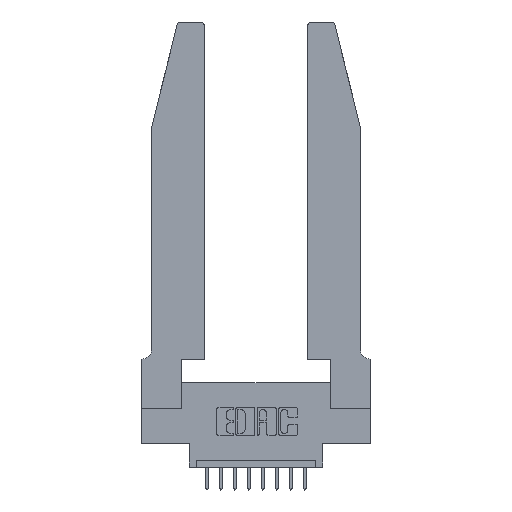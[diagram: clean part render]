
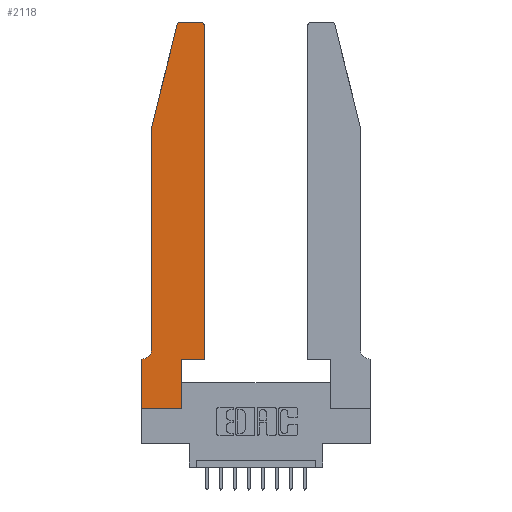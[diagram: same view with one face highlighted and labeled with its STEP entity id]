
A CAD part, top view. The second image highlights one B-rep face of the part: STEP entity #2118.
In plain terms, the highlighted planar face has unit normal (0, 0, 1).
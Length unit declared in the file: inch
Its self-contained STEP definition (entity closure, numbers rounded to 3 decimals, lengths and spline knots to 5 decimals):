
#182 = VERTEX_POINT ( 'NONE', #15368 ) ;
#187 = CARTESIAN_POINT ( 'NONE',  ( 0.284, 2.75, 0.37 ) ) ;
#546 = ORIENTED_EDGE ( 'NONE', *, *, #5395, .T. ) ;
#614 = CARTESIAN_POINT ( 'NONE',  ( 0., 0., 0.37 ) ) ;
#864 = VECTOR ( 'NONE', #15507, 39.37008 ) ;
#1088 = CARTESIAN_POINT ( 'NONE',  ( 0.2865, 0.35, 0.37 ) ) ;
#1105 = EDGE_CURVE ( 'NONE', #13346, #3585, #8174, .T. ) ;
#1202 = ORIENTED_EDGE ( 'NONE', *, *, #1105, .T. ) ;
#1531 = CARTESIAN_POINT ( 'NONE',  ( 0.0055, 0.42, 0.37 ) ) ;
#1691 = DIRECTION ( 'NONE',  ( 0., -1., 0. ) ) ;
#1773 = ORIENTED_EDGE ( 'NONE', *, *, #5691, .T. ) ;
#1904 = CARTESIAN_POINT ( 'NONE',  ( 0.4505, 0.35, 0.37 ) ) ;
#2008 = ORIENTED_EDGE ( 'NONE', *, *, #8542, .T. ) ;
#2118 = ADVANCED_FACE ( 'NONE', ( #8539 ), #2767, .T. ) ;
#2125 = CARTESIAN_POINT ( 'NONE',  ( 0.0755, 0.42, 0.37 ) ) ;
#2195 = LINE ( 'NONE', #2570, #8822 ) ;
#2570 = CARTESIAN_POINT ( 'NONE',  ( 0.0755, 2., 0.37 ) ) ;
#2637 = ORIENTED_EDGE ( 'NONE', *, *, #12434, .T. ) ;
#2767 = PLANE ( 'NONE',  #9166 ) ;
#3096 = VECTOR ( 'NONE', #4385, 39.37008 ) ;
#3184 = CIRCLE ( 'NONE', #5823, 0.03 ) ;
#3265 = CARTESIAN_POINT ( 'NONE',  ( 0.4505, 0.35, 0.37 ) ) ;
#3495 = LINE ( 'NONE', #8491, #9181 ) ;
#3585 = VERTEX_POINT ( 'NONE', #9422 ) ;
#3664 = EDGE_LOOP ( 'NONE', ( #3748, #1773, #546, #6605, #7809, #5660, #1202, #7066, #2008, #4316, #14859, #2637 ) ) ;
#3666 = DIRECTION ( 'NONE',  ( -0.239, -0.971, 0. ) ) ;
#3715 = AXIS2_PLACEMENT_3D ( 'NONE', #13348, #14555, #7445 ) ;
#3737 = CIRCLE ( 'NONE', #8466, 0.07 ) ;
#3748 = ORIENTED_EDGE ( 'NONE', *, *, #8498, .T. ) ;
#3868 = CARTESIAN_POINT ( 'NONE',  ( 0., 0.35, 0.37 ) ) ;
#4099 = VERTEX_POINT ( 'NONE', #9475 ) ;
#4208 = EDGE_CURVE ( 'NONE', #4697, #12306, #3737, .T. ) ;
#4245 = LINE ( 'NONE', #1088, #7446 ) ;
#4316 = ORIENTED_EDGE ( 'NONE', *, *, #6744, .T. ) ;
#4385 = DIRECTION ( 'NONE',  ( 0., 1., 0. ) ) ;
#4697 = VERTEX_POINT ( 'NONE', #2125 ) ;
#5004 = VERTEX_POINT ( 'NONE', #11173 ) ;
#5058 = DIRECTION ( 'NONE',  ( 1., 0., 0. ) ) ;
#5395 = EDGE_CURVE ( 'NONE', #5004, #12718, #2195, .T. ) ;
#5660 = ORIENTED_EDGE ( 'NONE', *, *, #11808, .T. ) ;
#5691 = EDGE_CURVE ( 'NONE', #8297, #5004, #8987, .T. ) ;
#5823 = AXIS2_PLACEMENT_3D ( 'NONE', #6659, #13746, #15062 ) ;
#6000 = LINE ( 'NONE', #6520, #6754 ) ;
#6298 = LINE ( 'NONE', #3265, #3096 ) ;
#6331 = VERTEX_POINT ( 'NONE', #1904 ) ;
#6490 = VECTOR ( 'NONE', #14520, 39.37008 ) ;
#6520 = CARTESIAN_POINT ( 'NONE',  ( 0.0755, 0.35, 0.37 ) ) ;
#6605 = ORIENTED_EDGE ( 'NONE', *, *, #6678, .T. ) ;
#6659 = CARTESIAN_POINT ( 'NONE',  ( 0.4205, 2.72, 0.37 ) ) ;
#6678 = EDGE_CURVE ( 'NONE', #12718, #4697, #3495, .T. ) ;
#6744 = EDGE_CURVE ( 'NONE', #14960, #6331, #7654, .T. ) ;
#6754 = VECTOR ( 'NONE', #10441, 39.37008 ) ;
#7066 = ORIENTED_EDGE ( 'NONE', *, *, #7527, .T. ) ;
#7139 = CARTESIAN_POINT ( 'NONE',  ( 0.4505, 0.35, 0.37 ) ) ;
#7445 = DIRECTION ( 'NONE',  ( 1., 0., 0. ) ) ;
#7446 = VECTOR ( 'NONE', #10774, 39.37008 ) ;
#7527 = EDGE_CURVE ( 'NONE', #3585, #182, #8007, .T. ) ;
#7654 = LINE ( 'NONE', #7139, #864 ) ;
#7809 = ORIENTED_EDGE ( 'NONE', *, *, #4208, .T. ) ;
#8007 = LINE ( 'NONE', #9731, #14950 ) ;
#8099 = CARTESIAN_POINT ( 'NONE',  ( 0.4205, 2.75, 0.37 ) ) ;
#8174 = LINE ( 'NONE', #614, #9327 ) ;
#8297 = VERTEX_POINT ( 'NONE', #187 ) ;
#8466 = AXIS2_PLACEMENT_3D ( 'NONE', #1531, #13561, #9989 ) ;
#8491 = CARTESIAN_POINT ( 'NONE',  ( 0.0755, 2., 0.37 ) ) ;
#8498 = EDGE_CURVE ( 'NONE', #10487, #8297, #10468, .T. ) ;
#8539 = FACE_OUTER_BOUND ( 'NONE', #3664, .T. ) ;
#8542 = EDGE_CURVE ( 'NONE', #182, #14960, #4245, .T. ) ;
#8667 = CARTESIAN_POINT ( 'NONE',  ( 0.0755, 2., 0.37 ) ) ;
#8822 = VECTOR ( 'NONE', #3666, 39.37008 ) ;
#8987 = CIRCLE ( 'NONE', #3715, 0.03 ) ;
#9056 = EDGE_CURVE ( 'NONE', #6331, #4099, #6298, .T. ) ;
#9166 = AXIS2_PLACEMENT_3D ( 'NONE', #3868, #10987, #14528 ) ;
#9181 = VECTOR ( 'NONE', #14277, 39.37008 ) ;
#9327 = VECTOR ( 'NONE', #1691, 39.37008 ) ;
#9422 = CARTESIAN_POINT ( 'NONE',  ( 0., 0., 0.37 ) ) ;
#9475 = CARTESIAN_POINT ( 'NONE',  ( 0.4505, 2.72, 0.37 ) ) ;
#9731 = CARTESIAN_POINT ( 'NONE',  ( 0., 0., 0.37 ) ) ;
#9989 = DIRECTION ( 'NONE',  ( -1., 0., 0. ) ) ;
#10076 = CARTESIAN_POINT ( 'NONE',  ( 0.0055, 0.35, 0.37 ) ) ;
#10441 = DIRECTION ( 'NONE',  ( -1., 0., 0. ) ) ;
#10468 = LINE ( 'NONE', #13071, #6490 ) ;
#10487 = VERTEX_POINT ( 'NONE', #8099 ) ;
#10774 = DIRECTION ( 'NONE',  ( 0., 1., 0. ) ) ;
#10987 = DIRECTION ( 'NONE',  ( 0., 0., 1. ) ) ;
#11173 = CARTESIAN_POINT ( 'NONE',  ( 0.25487, 2.72718, 0.37 ) ) ;
#11808 = EDGE_CURVE ( 'NONE', #12306, #13346, #6000, .T. ) ;
#11849 = CARTESIAN_POINT ( 'NONE',  ( 0., 0.35, 0.37 ) ) ;
#12306 = VERTEX_POINT ( 'NONE', #10076 ) ;
#12434 = EDGE_CURVE ( 'NONE', #4099, #10487, #3184, .T. ) ;
#12718 = VERTEX_POINT ( 'NONE', #8667 ) ;
#13071 = CARTESIAN_POINT ( 'NONE',  ( 0.2605, 2.75, 0.37 ) ) ;
#13117 = CARTESIAN_POINT ( 'NONE',  ( 0.2865, 0.35, 0.37 ) ) ;
#13346 = VERTEX_POINT ( 'NONE', #11849 ) ;
#13348 = CARTESIAN_POINT ( 'NONE',  ( 0.284, 2.72, 0.37 ) ) ;
#13561 = DIRECTION ( 'NONE',  ( 0., 0., -1. ) ) ;
#13746 = DIRECTION ( 'NONE',  ( 0., 0., 1. ) ) ;
#14277 = DIRECTION ( 'NONE',  ( 0., -1., 0. ) ) ;
#14520 = DIRECTION ( 'NONE',  ( -1., 0., 0. ) ) ;
#14528 = DIRECTION ( 'NONE',  ( 1., 0., 0. ) ) ;
#14555 = DIRECTION ( 'NONE',  ( 0., 0., 1. ) ) ;
#14859 = ORIENTED_EDGE ( 'NONE', *, *, #9056, .T. ) ;
#14950 = VECTOR ( 'NONE', #5058, 39.37008 ) ;
#14960 = VERTEX_POINT ( 'NONE', #13117 ) ;
#15062 = DIRECTION ( 'NONE',  ( 1., 0., 0. ) ) ;
#15368 = CARTESIAN_POINT ( 'NONE',  ( 0.2865, 0., 0.37 ) ) ;
#15507 = DIRECTION ( 'NONE',  ( 1., 0., 0. ) ) ;
